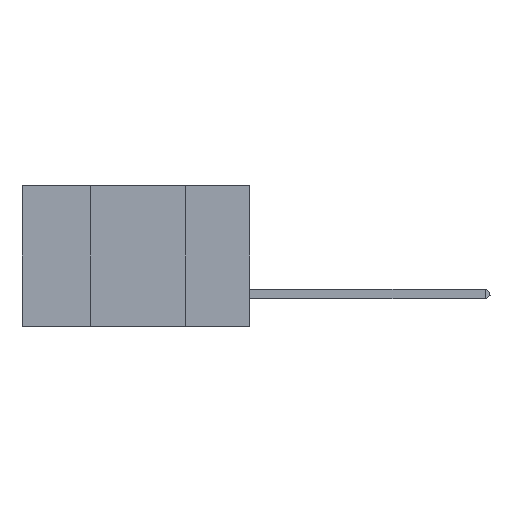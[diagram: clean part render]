
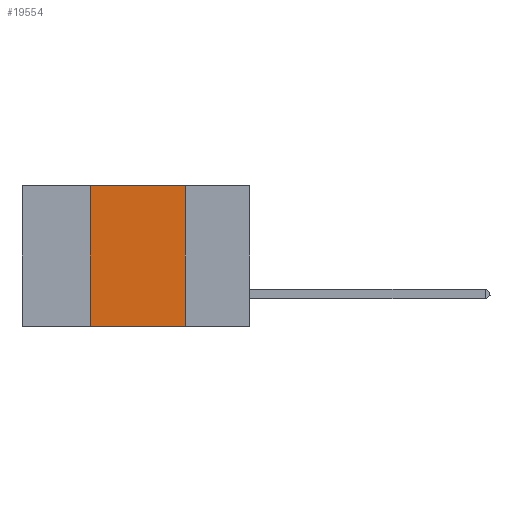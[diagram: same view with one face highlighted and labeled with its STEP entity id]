
A CAD part, left-side view. The second image highlights one B-rep face of the part: STEP entity #19554.
In plain terms, the highlighted planar face has unit normal (-1, 0, 0).
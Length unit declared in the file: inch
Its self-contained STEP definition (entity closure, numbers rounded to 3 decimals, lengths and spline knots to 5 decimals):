
#289 = ORIENTED_EDGE ( 'NONE', *, *, #24094, .T. ) ;
#516 = CARTESIAN_POINT ( 'NONE',  ( 0., 0.17, -0.37 ) ) ;
#994 = DIRECTION ( 'NONE',  ( 0., -1., 0. ) ) ;
#1447 = VECTOR ( 'NONE', #994, 39.37008 ) ;
#2320 = DIRECTION ( 'NONE',  ( 0., 0., 1. ) ) ;
#3457 = FACE_OUTER_BOUND ( 'NONE', #16158, .T. ) ;
#4256 = CARTESIAN_POINT ( 'NONE',  ( 0., 0.6, 0. ) ) ;
#5060 = DIRECTION ( 'NONE',  ( 1., 0., 0. ) ) ;
#5092 = EDGE_CURVE ( 'NONE', #24188, #13636, #16303, .T. ) ;
#5146 = CARTESIAN_POINT ( 'NONE',  ( 0., 0.42, -0.37 ) ) ;
#5712 = AXIS2_PLACEMENT_3D ( 'NONE', #14471, #5060, #7006 ) ;
#5920 = EDGE_CURVE ( 'NONE', #10155, #12821, #23678, .T. ) ;
#6226 = CARTESIAN_POINT ( 'NONE',  ( 0., 0.42, 0. ) ) ;
#7006 = DIRECTION ( 'NONE',  ( 0., 0., -1. ) ) ;
#7103 = DIRECTION ( 'NONE',  ( 0., 0., -1. ) ) ;
#8761 = CARTESIAN_POINT ( 'NONE',  ( 0., 0.42, 0. ) ) ;
#8984 = VECTOR ( 'NONE', #2320, 39.37008 ) ;
#9494 = ORIENTED_EDGE ( 'NONE', *, *, #5092, .F. ) ;
#10155 = VERTEX_POINT ( 'NONE', #17110 ) ;
#10354 = CARTESIAN_POINT ( 'NONE',  ( 0., 0.6, -0.37 ) ) ;
#11173 = ORIENTED_EDGE ( 'NONE', *, *, #5920, .F. ) ;
#12205 = VECTOR ( 'NONE', #7103, 39.37008 ) ;
#12544 = LINE ( 'NONE', #4256, #21937 ) ;
#12821 = VERTEX_POINT ( 'NONE', #516 ) ;
#13371 = DIRECTION ( 'NONE',  ( 0., -1., 0. ) ) ;
#13636 = VERTEX_POINT ( 'NONE', #8761 ) ;
#14471 = CARTESIAN_POINT ( 'NONE',  ( 0., 0.6, 0. ) ) ;
#15225 = LINE ( 'NONE', #10354, #1447 ) ;
#15720 = EDGE_CURVE ( 'NONE', #13636, #10155, #12544, .T. ) ;
#16158 = EDGE_LOOP ( 'NONE', ( #11173, #18687, #9494, #289 ) ) ;
#16303 = LINE ( 'NONE', #6226, #8984 ) ;
#16617 = PLANE ( 'NONE',  #5712 ) ;
#17110 = CARTESIAN_POINT ( 'NONE',  ( 0., 0.17, 0. ) ) ;
#18687 = ORIENTED_EDGE ( 'NONE', *, *, #15720, .F. ) ;
#19554 = ADVANCED_FACE ( 'NONE', ( #3457 ), #16617, .F. ) ;
#20332 = CARTESIAN_POINT ( 'NONE',  ( 0., 0.17, 0. ) ) ;
#21937 = VECTOR ( 'NONE', #13371, 39.37008 ) ;
#23678 = LINE ( 'NONE', #20332, #12205 ) ;
#24094 = EDGE_CURVE ( 'NONE', #24188, #12821, #15225, .T. ) ;
#24188 = VERTEX_POINT ( 'NONE', #5146 ) ;
